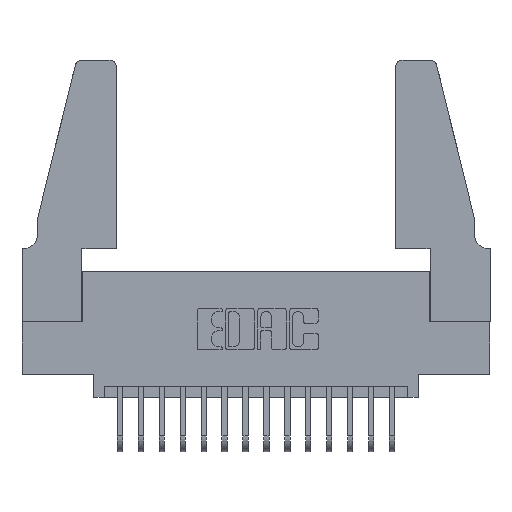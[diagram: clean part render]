
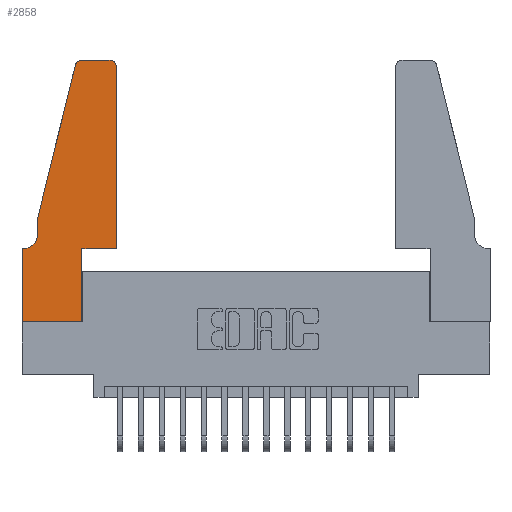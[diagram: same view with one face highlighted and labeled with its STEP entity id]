
A CAD part, top view. The second image highlights one B-rep face of the part: STEP entity #2858.
In plain terms, the highlighted planar face has unit normal (0, 0, 1).
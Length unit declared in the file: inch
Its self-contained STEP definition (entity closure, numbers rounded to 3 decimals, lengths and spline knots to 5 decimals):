
#82 = CARTESIAN_POINT ( 'NONE',  ( 0.4505, 0.35, 0.37 ) ) ;
#227 = LINE ( 'NONE', #2044, #7750 ) ;
#285 = EDGE_CURVE ( 'NONE', #2739, #1655, #4901, .T. ) ;
#375 = CARTESIAN_POINT ( 'NONE',  ( 0.4505, 1.22, 0.37 ) ) ;
#571 = CARTESIAN_POINT ( 'NONE',  ( 0., 0.35, 0.37 ) ) ;
#587 = CARTESIAN_POINT ( 'NONE',  ( 0.4205, 1.22, 0.37 ) ) ;
#856 = CARTESIAN_POINT ( 'NONE',  ( 0.2865, 0.35, 0.37 ) ) ;
#1231 = DIRECTION ( 'NONE',  ( -1., 0., 0. ) ) ;
#1256 = VERTEX_POINT ( 'NONE', #856 ) ;
#1267 = AXIS2_PLACEMENT_3D ( 'NONE', #10290, #6103, #7388 ) ;
#1346 = LINE ( 'NONE', #11325, #1820 ) ;
#1614 = VECTOR ( 'NONE', #1231, 39.37008 ) ;
#1655 = VERTEX_POINT ( 'NONE', #16594 ) ;
#1741 = EDGE_CURVE ( 'NONE', #17813, #9553, #2029, .T. ) ;
#1820 = VECTOR ( 'NONE', #4097, 39.37008 ) ;
#1968 = CARTESIAN_POINT ( 'NONE',  ( 0.4505, 0.35, 0.37 ) ) ;
#2005 = DIRECTION ( 'NONE',  ( -0.239, -0.971, 0. ) ) ;
#2029 = LINE ( 'NONE', #4077, #16038 ) ;
#2044 = CARTESIAN_POINT ( 'NONE',  ( 0.2865, 0.35, 0.37 ) ) ;
#2114 = DIRECTION ( 'NONE',  ( 1., 0., 0. ) ) ;
#2240 = DIRECTION ( 'NONE',  ( 1., 0., 0. ) ) ;
#2495 = DIRECTION ( 'NONE',  ( 0., -1., 0. ) ) ;
#2585 = LINE ( 'NONE', #1968, #10389 ) ;
#2672 = DIRECTION ( 'NONE',  ( 0., 0., 1. ) ) ;
#2739 = VERTEX_POINT ( 'NONE', #7754 ) ;
#2858 = ADVANCED_FACE ( 'NONE', ( #9625 ), #11872, .T. ) ;
#3072 = CARTESIAN_POINT ( 'NONE',  ( 0.284, 1.22, 0.37 ) ) ;
#3383 = CARTESIAN_POINT ( 'NONE',  ( 0.2605, 1.25, 0.37 ) ) ;
#3581 = VERTEX_POINT ( 'NONE', #3702 ) ;
#3591 = DIRECTION ( 'NONE',  ( 0., 1., 0. ) ) ;
#3702 = CARTESIAN_POINT ( 'NONE',  ( 0.284, 1.25, 0.37 ) ) ;
#4077 = CARTESIAN_POINT ( 'NONE',  ( 0.0755, 0.5, 0.37 ) ) ;
#4097 = DIRECTION ( 'NONE',  ( 0., -1., 0. ) ) ;
#4261 = VECTOR ( 'NONE', #4883, 39.37008 ) ;
#4579 = DIRECTION ( 'NONE',  ( 1., 0., 0. ) ) ;
#4883 = DIRECTION ( 'NONE',  ( -1., 0., 0. ) ) ;
#4892 = LINE ( 'NONE', #12724, #8336 ) ;
#4901 = CIRCLE ( 'NONE', #1267, 0.07 ) ;
#5161 = ORIENTED_EDGE ( 'NONE', *, *, #9668, .T. ) ;
#5236 = CARTESIAN_POINT ( 'NONE',  ( 0.4205, 1.25, 0.37 ) ) ;
#5375 = LINE ( 'NONE', #18290, #12549 ) ;
#5684 = ORIENTED_EDGE ( 'NONE', *, *, #7013, .T. ) ;
#5755 = EDGE_LOOP ( 'NONE', ( #5161, #5684, #9851, #14224, #12452, #15496, #15614, #16618, #11164, #15451, #17110, #18438 ) ) ;
#6103 = DIRECTION ( 'NONE',  ( 0., 0., -1. ) ) ;
#6225 = EDGE_CURVE ( 'NONE', #10532, #9686, #2585, .T. ) ;
#6621 = AXIS2_PLACEMENT_3D ( 'NONE', #3072, #13182, #4579 ) ;
#7013 = EDGE_CURVE ( 'NONE', #3581, #17813, #8267, .T. ) ;
#7037 = CARTESIAN_POINT ( 'NONE',  ( 0.4505, 0.35, 0.37 ) ) ;
#7388 = DIRECTION ( 'NONE',  ( -1., 0., 0. ) ) ;
#7750 = VECTOR ( 'NONE', #3591, 39.37008 ) ;
#7754 = CARTESIAN_POINT ( 'NONE',  ( 0.0755, 0.42, 0.37 ) ) ;
#7931 = VERTEX_POINT ( 'NONE', #571 ) ;
#8267 = CIRCLE ( 'NONE', #6621, 0.03 ) ;
#8336 = VECTOR ( 'NONE', #18351, 39.37008 ) ;
#9155 = CARTESIAN_POINT ( 'NONE',  ( 0.2865, 0., 0.37 ) ) ;
#9253 = EDGE_CURVE ( 'NONE', #18017, #1256, #227, .T. ) ;
#9320 = VERTEX_POINT ( 'NONE', #5236 ) ;
#9535 = CARTESIAN_POINT ( 'NONE',  ( 0., 0., 0.37 ) ) ;
#9551 = AXIS2_PLACEMENT_3D ( 'NONE', #587, #10919, #2114 ) ;
#9553 = VERTEX_POINT ( 'NONE', #13167 ) ;
#9625 = FACE_OUTER_BOUND ( 'NONE', #5755, .T. ) ;
#9668 = EDGE_CURVE ( 'NONE', #9320, #3581, #15675, .T. ) ;
#9686 = VERTEX_POINT ( 'NONE', #375 ) ;
#9813 = VERTEX_POINT ( 'NONE', #9535 ) ;
#9851 = ORIENTED_EDGE ( 'NONE', *, *, #1741, .T. ) ;
#10052 = EDGE_CURVE ( 'NONE', #1655, #7931, #13233, .T. ) ;
#10290 = CARTESIAN_POINT ( 'NONE',  ( 0.0055, 0.42, 0.37 ) ) ;
#10389 = VECTOR ( 'NONE', #12179, 39.37008 ) ;
#10532 = VERTEX_POINT ( 'NONE', #7037 ) ;
#10919 = DIRECTION ( 'NONE',  ( 0., 0., 1. ) ) ;
#11164 = ORIENTED_EDGE ( 'NONE', *, *, #9253, .T. ) ;
#11325 = CARTESIAN_POINT ( 'NONE',  ( 0., 0., 0.37 ) ) ;
#11528 = CARTESIAN_POINT ( 'NONE',  ( 0.25487, 1.22718, 0.37 ) ) ;
#11872 = PLANE ( 'NONE',  #12442 ) ;
#11878 = VECTOR ( 'NONE', #17503, 39.37008 ) ;
#12152 = CIRCLE ( 'NONE', #9551, 0.03 ) ;
#12179 = DIRECTION ( 'NONE',  ( 0., 1., 0. ) ) ;
#12303 = LINE ( 'NONE', #82, #11878 ) ;
#12442 = AXIS2_PLACEMENT_3D ( 'NONE', #18383, #2672, #2240 ) ;
#12452 = ORIENTED_EDGE ( 'NONE', *, *, #285, .T. ) ;
#12549 = VECTOR ( 'NONE', #2495, 39.37008 ) ;
#12724 = CARTESIAN_POINT ( 'NONE',  ( 0., 0., 0.37 ) ) ;
#13167 = CARTESIAN_POINT ( 'NONE',  ( 0.0755, 0.5, 0.37 ) ) ;
#13182 = DIRECTION ( 'NONE',  ( 0., 0., 1. ) ) ;
#13233 = LINE ( 'NONE', #18476, #1614 ) ;
#14224 = ORIENTED_EDGE ( 'NONE', *, *, #16540, .T. ) ;
#14666 = EDGE_CURVE ( 'NONE', #9686, #9320, #12152, .T. ) ;
#15451 = ORIENTED_EDGE ( 'NONE', *, *, #16806, .T. ) ;
#15496 = ORIENTED_EDGE ( 'NONE', *, *, #10052, .T. ) ;
#15614 = ORIENTED_EDGE ( 'NONE', *, *, #16545, .T. ) ;
#15675 = LINE ( 'NONE', #3383, #4261 ) ;
#16038 = VECTOR ( 'NONE', #2005, 39.37008 ) ;
#16540 = EDGE_CURVE ( 'NONE', #9553, #2739, #5375, .T. ) ;
#16545 = EDGE_CURVE ( 'NONE', #7931, #9813, #1346, .T. ) ;
#16586 = EDGE_CURVE ( 'NONE', #9813, #18017, #4892, .T. ) ;
#16594 = CARTESIAN_POINT ( 'NONE',  ( 0.0055, 0.35, 0.37 ) ) ;
#16618 = ORIENTED_EDGE ( 'NONE', *, *, #16586, .T. ) ;
#16806 = EDGE_CURVE ( 'NONE', #1256, #10532, #12303, .T. ) ;
#17110 = ORIENTED_EDGE ( 'NONE', *, *, #6225, .T. ) ;
#17503 = DIRECTION ( 'NONE',  ( 1., 0., 0. ) ) ;
#17813 = VERTEX_POINT ( 'NONE', #11528 ) ;
#18017 = VERTEX_POINT ( 'NONE', #9155 ) ;
#18290 = CARTESIAN_POINT ( 'NONE',  ( 0.0755, 0.5, 0.37 ) ) ;
#18351 = DIRECTION ( 'NONE',  ( 1., 0., 0. ) ) ;
#18383 = CARTESIAN_POINT ( 'NONE',  ( 0., 0.35, 0.37 ) ) ;
#18438 = ORIENTED_EDGE ( 'NONE', *, *, #14666, .T. ) ;
#18476 = CARTESIAN_POINT ( 'NONE',  ( 0.0755, 0.35, 0.37 ) ) ;
